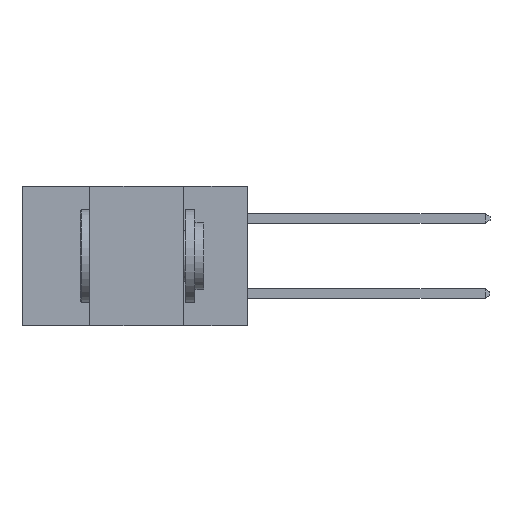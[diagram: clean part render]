
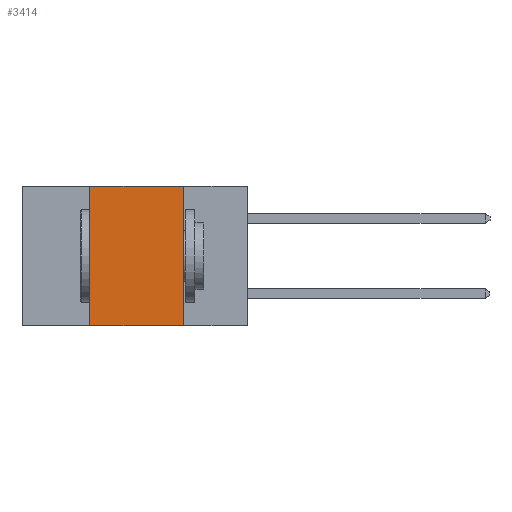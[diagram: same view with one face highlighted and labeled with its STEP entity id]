
A CAD part, left-side view. The second image highlights one B-rep face of the part: STEP entity #3414.
In plain terms, the highlighted planar face has unit normal (-1, 0, 0).
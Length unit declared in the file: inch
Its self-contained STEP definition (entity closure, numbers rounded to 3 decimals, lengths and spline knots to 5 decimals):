
#920 = VERTEX_POINT ( 'NONE', #15598 ) ;
#1065 = VECTOR ( 'NONE', #17669, 39.37008 ) ;
#1450 = DIRECTION ( 'NONE',  ( 0., 0., -1. ) ) ;
#2177 = ORIENTED_EDGE ( 'NONE', *, *, #12972, .F. ) ;
#2201 = LINE ( 'NONE', #12333, #16703 ) ;
#2652 = ORIENTED_EDGE ( 'NONE', *, *, #6577, .F. ) ;
#3144 = ORIENTED_EDGE ( 'NONE', *, *, #10972, .T. ) ;
#3414 = ADVANCED_FACE ( 'NONE', ( #16253 ), #7667, .F. ) ;
#3614 = EDGE_LOOP ( 'NONE', ( #18075, #2177, #2652, #3144 ) ) ;
#4198 = CARTESIAN_POINT ( 'NONE',  ( 0., 0.6, 0. ) ) ;
#4817 = DIRECTION ( 'NONE',  ( 0., 0., 1. ) ) ;
#4931 = DIRECTION ( 'NONE',  ( 0., 0., -1. ) ) ;
#4976 = DIRECTION ( 'NONE',  ( 1., 0., 0. ) ) ;
#5397 = LINE ( 'NONE', #12619, #13296 ) ;
#6577 = EDGE_CURVE ( 'NONE', #9280, #12481, #5397, .T. ) ;
#7421 = CARTESIAN_POINT ( 'NONE',  ( 0., 0.6, 0. ) ) ;
#7667 = PLANE ( 'NONE',  #8141 ) ;
#8141 = AXIS2_PLACEMENT_3D ( 'NONE', #7421, #4976, #4931 ) ;
#8152 = LINE ( 'NONE', #8405, #1065 ) ;
#8405 = CARTESIAN_POINT ( 'NONE',  ( 0., 0.6, -0.37 ) ) ;
#8821 = LINE ( 'NONE', #4198, #16134 ) ;
#9280 = VERTEX_POINT ( 'NONE', #15652 ) ;
#9969 = CARTESIAN_POINT ( 'NONE',  ( 0., 0.17, -0.37 ) ) ;
#10972 = EDGE_CURVE ( 'NONE', #9280, #14656, #8152, .T. ) ;
#12333 = CARTESIAN_POINT ( 'NONE',  ( 0., 0.17, 0. ) ) ;
#12481 = VERTEX_POINT ( 'NONE', #15546 ) ;
#12619 = CARTESIAN_POINT ( 'NONE',  ( 0., 0.42, 0. ) ) ;
#12972 = EDGE_CURVE ( 'NONE', #12481, #920, #8821, .T. ) ;
#13296 = VECTOR ( 'NONE', #4817, 39.37008 ) ;
#14656 = VERTEX_POINT ( 'NONE', #9969 ) ;
#15059 = DIRECTION ( 'NONE',  ( 0., -1., 0. ) ) ;
#15546 = CARTESIAN_POINT ( 'NONE',  ( 0., 0.42, 0. ) ) ;
#15598 = CARTESIAN_POINT ( 'NONE',  ( 0., 0.17, 0. ) ) ;
#15652 = CARTESIAN_POINT ( 'NONE',  ( 0., 0.42, -0.37 ) ) ;
#16134 = VECTOR ( 'NONE', #15059, 39.37008 ) ;
#16253 = FACE_OUTER_BOUND ( 'NONE', #3614, .T. ) ;
#16703 = VECTOR ( 'NONE', #1450, 39.37008 ) ;
#16818 = EDGE_CURVE ( 'NONE', #920, #14656, #2201, .T. ) ;
#17669 = DIRECTION ( 'NONE',  ( 0., -1., 0. ) ) ;
#18075 = ORIENTED_EDGE ( 'NONE', *, *, #16818, .F. ) ;
